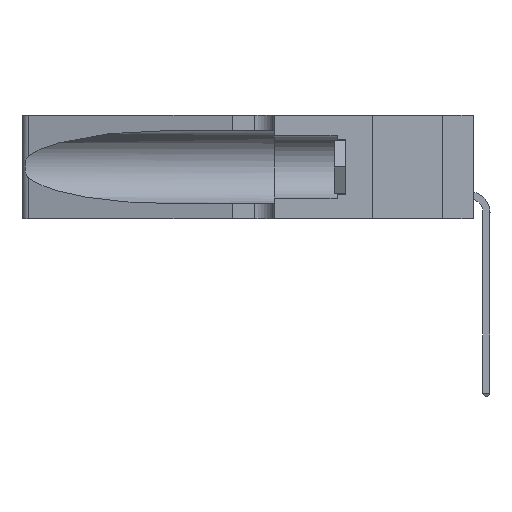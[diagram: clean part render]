
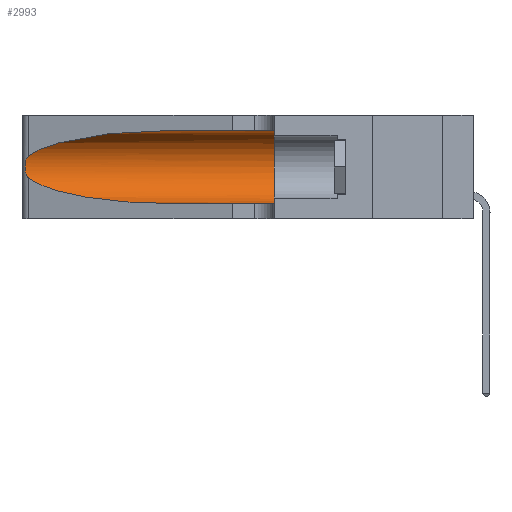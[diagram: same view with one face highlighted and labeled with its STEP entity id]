
A CAD part, left-side view. The second image highlights one B-rep face of the part: STEP entity #2993.
In plain terms, the highlighted cylindrical face has radius 3.308 mm (diameter 6.617 mm), a partial arc.
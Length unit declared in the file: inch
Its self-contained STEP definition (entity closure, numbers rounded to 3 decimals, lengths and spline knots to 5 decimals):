
#1087 = CARTESIAN_POINT ( 'NONE',  ( 0.25487, 1.22718, 0.14631 ) ) ;
#1103 = FACE_OUTER_BOUND ( 'NONE', #6265, .T. ) ;
#1240 = CARTESIAN_POINT ( 'NONE',  ( 0.26075, 1.23896, 0.178 ) ) ;
#1690 = ORIENTED_EDGE ( 'NONE', *, *, #15785, .F. ) ;
#1729 = CARTESIAN_POINT ( 'NONE',  ( 0.25487, 1.22718, 0.22369 ) ) ;
#1808 = CARTESIAN_POINT ( 'NONE',  ( 0.1305, 0.35, 0.05475 ) ) ;
#2136 = VECTOR ( 'NONE', #27078, 39.37008 ) ;
#2993 = ADVANCED_FACE ( 'NONE', ( #1103 ), #35426, .F. ) ;
#3687 = AXIS2_PLACEMENT_3D ( 'NONE', #23223, #33752, #17997 ) ;
#3783 = VERTEX_POINT ( 'NONE', #13045 ) ;
#4495 = CARTESIAN_POINT ( 'NONE',  ( 0.26075, 1.23896, 0.19203 ) ) ;
#4957 = CARTESIAN_POINT ( 'NONE',  ( 0.26018, 1.23835, 0.19895 ) ) ;
#6265 = EDGE_LOOP ( 'NONE', ( #22587, #29886, #35645, #43002, #1690, #38869 ) ) ;
#6329 = EDGE_CURVE ( 'NONE', #28093, #3783, #19589, .T. ) ;
#8433 = CARTESIAN_POINT ( 'NONE',  ( 0.25787, 1.23484, 0.2124 ) ) ;
#11113 = LINE ( 'NONE', #26887, #37867 ) ;
#11264 = CARTESIAN_POINT ( 'NONE',  ( 0.26017, 1.23833, 0.17102 ) ) ;
#12056 = CARTESIAN_POINT ( 'NONE',  ( 0.18966, 0.96281, 0.31525 ) ) ;
#13045 = CARTESIAN_POINT ( 'NONE',  ( 0.25487, 1.22718, 0.14631 ) ) ;
#13525 = LINE ( 'NONE', #40481, #2136 ) ;
#15218 = CARTESIAN_POINT ( 'NONE',  ( 0.25856, 1.23593, 0.16098 ) ) ;
#15565 = CARTESIAN_POINT ( 'NONE',  ( 0.2373, 1.15595, 0.28018 ) ) ;
#15785 = EDGE_CURVE ( 'NONE', #38605, #16962, #18505, .T. ) ;
#16278 = DIRECTION ( 'NONE',  ( 0., 0., -1. ) ) ;
#16383 = EDGE_CURVE ( 'NONE', #21603, #38605, #13525, .T. ) ;
#16962 = VERTEX_POINT ( 'NONE', #1808 ) ;
#17553 = VERTEX_POINT ( 'NONE', #40727 ) ;
#17997 = DIRECTION ( 'NONE',  ( 0., 0., 1. ) ) ;
#18505 = CIRCLE ( 'NONE', #3687, 0.13025 ) ;
#18574 = CARTESIAN_POINT ( 'NONE',  ( 0.25854, 1.2359, 0.20912 ) ) ;
#18681 = CARTESIAN_POINT ( 'NONE',  ( 0.1305, 0.72297, 0.31525 ) ) ;
#19574 = EDGE_CURVE ( 'NONE', #3783, #17553, #44717, .T. ) ;
#19589 = B_SPLINE_CURVE_WITH_KNOTS ( 'NONE', 3,
 ( #36102, #21744, #39445, #8433, #18574, #4957, #4495, #1240, #11264, #15218, #21889, #39143, #22048, #1087 ),
 .UNSPECIFIED., .F., .F.,
 ( 4, 2, 2, 2, 2, 2, 4 ),
 ( 0., 0.00027, 0.00053, 0.00107, 0.0016, 0.00187, 0.00214 ),
 .UNSPECIFIED. ) ;
#20592 = CARTESIAN_POINT ( 'NONE',  ( 0.1305, 0.72297, 0.05475 ) ) ;
#20729 = CARTESIAN_POINT ( 'NONE',  ( 0.25487, 1.22718, 0.14631 ) ) ;
#21603 = VERTEX_POINT ( 'NONE', #18681 ) ;
#21744 = CARTESIAN_POINT ( 'NONE',  ( 0.25555, 1.22994, 0.2215 ) ) ;
#21889 = CARTESIAN_POINT ( 'NONE',  ( 0.25789, 1.23486, 0.15765 ) ) ;
#22048 = CARTESIAN_POINT ( 'NONE',  ( 0.25555, 1.22993, 0.14849 ) ) ;
#22392 = CARTESIAN_POINT ( 'NONE',  ( 0.1305, 0.35, 0.31525 ) ) ;
#22587 = ORIENTED_EDGE ( 'NONE', *, *, #43088, .T. ) ;
#23223 = CARTESIAN_POINT ( 'NONE',  ( 0.1305, 0.35, 0.185 ) ) ;
#23962 = CARTESIAN_POINT ( 'NONE',  ( 0.18966, 0.96281, 0.05475 ) ) ;
#26887 = CARTESIAN_POINT ( 'NONE',  ( 0.1305, 1.61858, 0.05475 ) ) ;
#27078 = DIRECTION ( 'NONE',  ( 0., -1., 0. ) ) ;
#27109 = DIRECTION ( 'NONE',  ( 0., -1., 0. ) ) ;
#28093 = VERTEX_POINT ( 'NONE', #29468 ) ;
#29429 = CARTESIAN_POINT ( 'NONE',  ( 0.1305, 0.72297, 0.31525 ) ) ;
#29468 = CARTESIAN_POINT ( 'NONE',  ( 0.25487, 1.22718, 0.22369 ) ) ;
#29886 = ORIENTED_EDGE ( 'NONE', *, *, #6329, .T. ) ;
#30361 = DIRECTION ( 'NONE',  ( 0., -1., 0. ) ) ;
#30428 = CARTESIAN_POINT ( 'NONE',  ( 0.1305, 1.61858, 0.185 ) ) ;
#31806 = EDGE_CURVE ( 'NONE', #17553, #16962, #11113, .T. ) ;
#33752 = DIRECTION ( 'NONE',  ( 0., 1., 0. ) ) ;
#34349 = CARTESIAN_POINT ( 'NONE',  ( 0.2373, 1.15595, 0.08982 ) ) ;
#35426 = CYLINDRICAL_SURFACE ( 'NONE', #43888, 0.13025 ) ;
#35645 = ORIENTED_EDGE ( 'NONE', *, *, #19574, .T. ) ;
#36102 = CARTESIAN_POINT ( 'NONE',  ( 0.25487, 1.22718, 0.22369 ) ) ;
#37867 = VECTOR ( 'NONE', #30361, 39.37008 ) ;
#38605 = VERTEX_POINT ( 'NONE', #22392 ) ;
#38869 = ORIENTED_EDGE ( 'NONE', *, *, #16383, .F. ) ;
#39143 = CARTESIAN_POINT ( 'NONE',  ( 0.25639, 1.23186, 0.15144 ) ) ;
#39445 = CARTESIAN_POINT ( 'NONE',  ( 0.25639, 1.23184, 0.21858 ) ) ;
#40481 = CARTESIAN_POINT ( 'NONE',  ( 0.1305, 1.61858, 0.31525 ) ) ;
#40727 = CARTESIAN_POINT ( 'NONE',  ( 0.1305, 0.72297, 0.05475 ) ) ;
#43002 = ORIENTED_EDGE ( 'NONE', *, *, #31806, .T. ) ;
#43088 = EDGE_CURVE ( 'NONE', #21603, #28093, #43314, .T. ) ;
#43314 =( BOUNDED_CURVE ( )  B_SPLINE_CURVE ( 3, ( #29429, #12056, #15565, #1729 ),
 .UNSPECIFIED., .F., .T. ) 
 B_SPLINE_CURVE_WITH_KNOTS ( ( 4, 4 ),
 ( 1.5708, 2.84003 ),
 .UNSPECIFIED. ) 
 CURVE ( )  GEOMETRIC_REPRESENTATION_ITEM ( )  RATIONAL_B_SPLINE_CURVE ( ( 1., 0.87, 0.87, 1. ) ) 
 REPRESENTATION_ITEM ( '' )  );
#43888 = AXIS2_PLACEMENT_3D ( 'NONE', #30428, #27109, #16278 ) ;
#44717 =( BOUNDED_CURVE ( )  B_SPLINE_CURVE ( 3, ( #20729, #34349, #23962, #20592 ),
 .UNSPECIFIED., .F., .T. ) 
 B_SPLINE_CURVE_WITH_KNOTS ( ( 4, 4 ),
 ( 3.44316, 4.71239 ),
 .UNSPECIFIED. ) 
 CURVE ( )  GEOMETRIC_REPRESENTATION_ITEM ( )  RATIONAL_B_SPLINE_CURVE ( ( 1., 0.87, 0.87, 1. ) ) 
 REPRESENTATION_ITEM ( '' )  );
